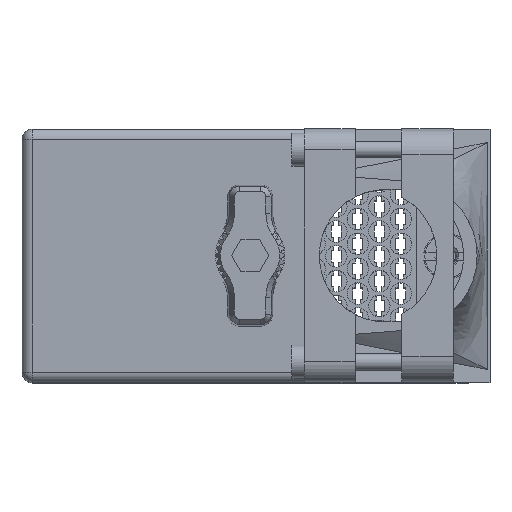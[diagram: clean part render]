
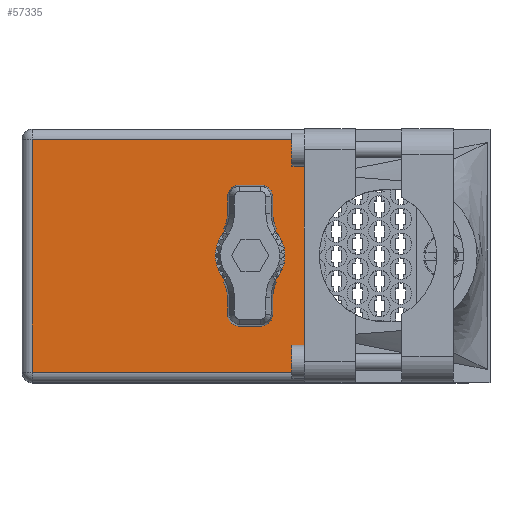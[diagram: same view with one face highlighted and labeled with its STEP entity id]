
A CAD part, top view. The second image highlights one B-rep face of the part: STEP entity #57335.
In plain terms, the highlighted face is planar.
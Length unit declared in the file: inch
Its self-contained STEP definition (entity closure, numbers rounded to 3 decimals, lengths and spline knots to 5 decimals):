
#5765 = EDGE_CURVE ( 'NONE', #46384, #23456, #30483, .T. ) ;
#7645 = ORIENTED_EDGE ( 'NONE', *, *, #5765, .T. ) ;
#9129 = CARTESIAN_POINT ( 'NONE',  ( 1.3775, 2.03, -0.765 ) ) ;
#9221 = VECTOR ( 'NONE', #94964, 39.37008 ) ;
#9600 = DIRECTION ( 'NONE',  ( 0., 0., 1. ) ) ;
#10448 = FACE_OUTER_BOUND ( 'NONE', #72379, .T. ) ;
#12573 = CIRCLE ( 'NONE', #86442, 0.1015 ) ;
#13670 = VECTOR ( 'NONE', #104766, 39.37008 ) ;
#14289 = LINE ( 'NONE', #107009, #53560 ) ;
#16459 = AXIS2_PLACEMENT_3D ( 'NONE', #79089, #35176, #45381 ) ;
#20958 = EDGE_CURVE ( 'NONE', #22928, #46384, #57187, .T. ) ;
#22928 = VERTEX_POINT ( 'NONE', #53705 ) ;
#23456 = VERTEX_POINT ( 'NONE', #30504 ) ;
#25088 = ORIENTED_EDGE ( 'NONE', *, *, #110416, .T. ) ;
#29716 = CARTESIAN_POINT ( 'NONE',  ( 1.3775, 2.03, -0.765 ) ) ;
#30483 = LINE ( 'NONE', #95731, #68335 ) ;
#30504 = CARTESIAN_POINT ( 'NONE',  ( 0.062, 2.03, -0.062 ) ) ;
#31549 = EDGE_LOOP ( 'NONE', ( #44175, #53454 ) ) ;
#34265 = CIRCLE ( 'NONE', #46804, 0.1015 ) ;
#35176 = DIRECTION ( 'NONE',  ( 0., 1., 0. ) ) ;
#41146 = EDGE_CURVE ( 'NONE', #22928, #67734, #108286, .T. ) ;
#42963 = DIRECTION ( 'NONE',  ( 0., 0., 1. ) ) ;
#44175 = ORIENTED_EDGE ( 'NONE', *, *, #67721, .F. ) ;
#44625 = PLANE ( 'NONE',  #16459 ) ;
#45381 = DIRECTION ( 'NONE',  ( 0., 0., 1. ) ) ;
#46384 = VERTEX_POINT ( 'NONE', #65216 ) ;
#46804 = AXIS2_PLACEMENT_3D ( 'NONE', #29716, #56546, #90288 ) ;
#52410 = DIRECTION ( 'NONE',  ( 0., 1., 0. ) ) ;
#53454 = ORIENTED_EDGE ( 'NONE', *, *, #60612, .F. ) ;
#53560 = VECTOR ( 'NONE', #89902, 39.37008 ) ;
#53705 = CARTESIAN_POINT ( 'NONE',  ( 1.705, 2.03, -1.468 ) ) ;
#54824 = CARTESIAN_POINT ( 'NONE',  ( 1.3775, 2.03, -0.8665 ) ) ;
#56546 = DIRECTION ( 'NONE',  ( 0., 1., 0. ) ) ;
#57187 = LINE ( 'NONE', #105531, #13670 ) ;
#57335 = ADVANCED_FACE ( 'NONE', ( #10448, #83711 ), #44625, .T. ) ;
#60612 = EDGE_CURVE ( 'NONE', #99546, #91919, #34265, .T. ) ;
#65216 = CARTESIAN_POINT ( 'NONE',  ( 0.062, 2.03, -1.468 ) ) ;
#67721 = EDGE_CURVE ( 'NONE', #91919, #99546, #12573, .T. ) ;
#67734 = VERTEX_POINT ( 'NONE', #78177 ) ;
#68335 = VECTOR ( 'NONE', #9600, 39.37008 ) ;
#72379 = EDGE_LOOP ( 'NONE', ( #7645, #25088, #112219, #95496 ) ) ;
#78177 = CARTESIAN_POINT ( 'NONE',  ( 1.705, 2.03, -0.062 ) ) ;
#79089 = CARTESIAN_POINT ( 'NONE',  ( 0., 2.03, -1.53 ) ) ;
#83711 = FACE_BOUND ( 'NONE', #31549, .T. ) ;
#86442 = AXIS2_PLACEMENT_3D ( 'NONE', #9129, #52410, #42963 ) ;
#89902 = DIRECTION ( 'NONE',  ( 1., 0., 0. ) ) ;
#90288 = DIRECTION ( 'NONE',  ( 0., 0., 1. ) ) ;
#91919 = VERTEX_POINT ( 'NONE', #100026 ) ;
#94964 = DIRECTION ( 'NONE',  ( 0., 0., 1. ) ) ;
#95496 = ORIENTED_EDGE ( 'NONE', *, *, #20958, .T. ) ;
#95731 = CARTESIAN_POINT ( 'NONE',  ( 0.062, 2.03, -1.53 ) ) ;
#99546 = VERTEX_POINT ( 'NONE', #54824 ) ;
#100026 = CARTESIAN_POINT ( 'NONE',  ( 1.3775, 2.03, -0.6635 ) ) ;
#102977 = CARTESIAN_POINT ( 'NONE',  ( 1.705, 2.03, -1.53 ) ) ;
#104766 = DIRECTION ( 'NONE',  ( -1., 0., 0. ) ) ;
#105531 = CARTESIAN_POINT ( 'NONE',  ( 0., 2.03, -1.468 ) ) ;
#107009 = CARTESIAN_POINT ( 'NONE',  ( 1.705, 2.03, -0.062 ) ) ;
#108286 = LINE ( 'NONE', #102977, #9221 ) ;
#110416 = EDGE_CURVE ( 'NONE', #23456, #67734, #14289, .T. ) ;
#112219 = ORIENTED_EDGE ( 'NONE', *, *, #41146, .F. ) ;
